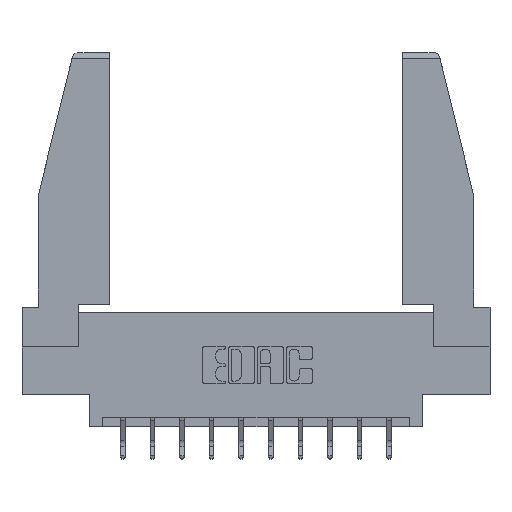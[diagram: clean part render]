
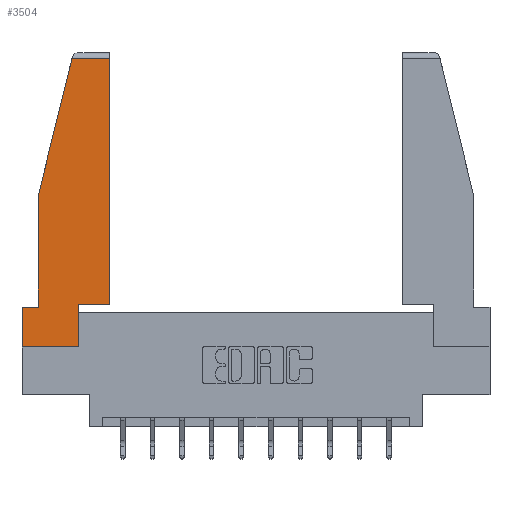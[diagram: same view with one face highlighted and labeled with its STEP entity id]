
A CAD part, top view. The second image highlights one B-rep face of the part: STEP entity #3504.
In plain terms, the highlighted planar face has unit normal (0, 0, 1).
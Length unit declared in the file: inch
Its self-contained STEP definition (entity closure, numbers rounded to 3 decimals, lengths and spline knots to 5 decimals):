
#660 = CARTESIAN_POINT ( 'NONE',  ( 0., 1.52, 0. ) ) ;
#703 = EDGE_CURVE ( 'NONE', #13000, #8001, #8081, .T. ) ;
#913 = CARTESIAN_POINT ( 'NONE',  ( 0.086, 0.21, 0. ) ) ;
#945 = AXIS2_PLACEMENT_3D ( 'NONE', #13486, #1005, #4476 ) ;
#990 = VERTEX_POINT ( 'NONE', #6314 ) ;
#1005 = DIRECTION ( 'NONE',  ( 0., 0., 1. ) ) ;
#1070 = CARTESIAN_POINT ( 'NONE',  ( 0.461, 0.223, 0. ) ) ;
#1220 = DIRECTION ( 'NONE',  ( 1., 0., 0. ) ) ;
#1303 = VECTOR ( 'NONE', #13057, 39.37008 ) ;
#1536 = CARTESIAN_POINT ( 'NONE',  ( 0., 0., 0. ) ) ;
#1809 = LINE ( 'NONE', #13402, #13564 ) ;
#2137 = ORIENTED_EDGE ( 'NONE', *, *, #10737, .T. ) ;
#2247 = ORIENTED_EDGE ( 'NONE', *, *, #11042, .T. ) ;
#2599 = EDGE_CURVE ( 'NONE', #6331, #10988, #8358, .T. ) ;
#3091 = CARTESIAN_POINT ( 'NONE',  ( 0.2636, 1.52, 0. ) ) ;
#3504 = ADVANCED_FACE ( 'NONE', ( #8229 ), #9974, .T. ) ;
#3506 = VERTEX_POINT ( 'NONE', #3091 ) ;
#3553 = DIRECTION ( 'NONE',  ( 0., -1., 0. ) ) ;
#4240 = DIRECTION ( 'NONE',  ( 0., 1., 0. ) ) ;
#4410 = LINE ( 'NONE', #660, #14593 ) ;
#4476 = DIRECTION ( 'NONE',  ( 1., 0., 0. ) ) ;
#4838 = LINE ( 'NONE', #5781, #12177 ) ;
#4849 = LINE ( 'NONE', #7688, #7523 ) ;
#4911 = CARTESIAN_POINT ( 'NONE',  ( 0.297, 0.223, 0. ) ) ;
#5062 = CARTESIAN_POINT ( 'NONE',  ( 0., 0.21, 0. ) ) ;
#5079 = CARTESIAN_POINT ( 'NONE',  ( 0.297, 0., 0. ) ) ;
#5183 = LINE ( 'NONE', #5062, #8581 ) ;
#5534 = VECTOR ( 'NONE', #4240, 39.37008 ) ;
#5781 = CARTESIAN_POINT ( 'NONE',  ( 0.086, 0.8, 0. ) ) ;
#5791 = CARTESIAN_POINT ( 'NONE',  ( 0., 0.21, 0. ) ) ;
#6314 = CARTESIAN_POINT ( 'NONE',  ( 0.461, 1.52, 0. ) ) ;
#6331 = VERTEX_POINT ( 'NONE', #913 ) ;
#6645 = EDGE_CURVE ( 'NONE', #990, #3506, #4410, .T. ) ;
#6963 = DIRECTION ( 'NONE',  ( -1., 0., 0. ) ) ;
#7411 = ORIENTED_EDGE ( 'NONE', *, *, #10278, .T. ) ;
#7464 = VECTOR ( 'NONE', #6963, 39.37008 ) ;
#7523 = VECTOR ( 'NONE', #14342, 39.37008 ) ;
#7688 = CARTESIAN_POINT ( 'NONE',  ( 0.297, 0., 0. ) ) ;
#7828 = ORIENTED_EDGE ( 'NONE', *, *, #703, .T. ) ;
#8001 = VERTEX_POINT ( 'NONE', #1070 ) ;
#8043 = CARTESIAN_POINT ( 'NONE',  ( 0.297, 0.223, 0. ) ) ;
#8050 = LINE ( 'NONE', #11100, #5534 ) ;
#8081 = LINE ( 'NONE', #8043, #9873 ) ;
#8229 = FACE_OUTER_BOUND ( 'NONE', #10277, .T. ) ;
#8358 = LINE ( 'NONE', #5791, #7464 ) ;
#8581 = VECTOR ( 'NONE', #13192, 39.37008 ) ;
#8612 = DIRECTION ( 'NONE',  ( -1., 0., 0. ) ) ;
#8626 = CARTESIAN_POINT ( 'NONE',  ( 0., 0., 0. ) ) ;
#9126 = LINE ( 'NONE', #8626, #1303 ) ;
#9383 = CARTESIAN_POINT ( 'NONE',  ( 0., 0.21, 0. ) ) ;
#9873 = VECTOR ( 'NONE', #1220, 39.37008 ) ;
#9974 = PLANE ( 'NONE',  #945 ) ;
#10083 = VERTEX_POINT ( 'NONE', #11095 ) ;
#10277 = EDGE_LOOP ( 'NONE', ( #2247, #14569, #14651, #2137, #14361, #12227, #13773, #7411, #7828 ) ) ;
#10278 = EDGE_CURVE ( 'NONE', #10771, #13000, #4849, .T. ) ;
#10737 = EDGE_CURVE ( 'NONE', #10083, #6331, #4838, .T. ) ;
#10755 = EDGE_CURVE ( 'NONE', #13445, #10771, #9126, .T. ) ;
#10771 = VERTEX_POINT ( 'NONE', #5079 ) ;
#10970 = EDGE_CURVE ( 'NONE', #10988, #13445, #5183, .T. ) ;
#10988 = VERTEX_POINT ( 'NONE', #9383 ) ;
#11042 = EDGE_CURVE ( 'NONE', #8001, #990, #8050, .T. ) ;
#11095 = CARTESIAN_POINT ( 'NONE',  ( 0.086, 0.8, 0. ) ) ;
#11098 = EDGE_CURVE ( 'NONE', #3506, #10083, #1809, .T. ) ;
#11100 = CARTESIAN_POINT ( 'NONE',  ( 0.461, 0.223, 0. ) ) ;
#12177 = VECTOR ( 'NONE', #3553, 39.37008 ) ;
#12227 = ORIENTED_EDGE ( 'NONE', *, *, #10970, .T. ) ;
#13000 = VERTEX_POINT ( 'NONE', #4911 ) ;
#13057 = DIRECTION ( 'NONE',  ( 1., 0., 0. ) ) ;
#13192 = DIRECTION ( 'NONE',  ( 0., -1., 0. ) ) ;
#13402 = CARTESIAN_POINT ( 'NONE',  ( 0.271, 1.55, 0. ) ) ;
#13445 = VERTEX_POINT ( 'NONE', #1536 ) ;
#13486 = CARTESIAN_POINT ( 'NONE',  ( 0., 0., 0. ) ) ;
#13564 = VECTOR ( 'NONE', #14589, 39.37008 ) ;
#13773 = ORIENTED_EDGE ( 'NONE', *, *, #10755, .T. ) ;
#14342 = DIRECTION ( 'NONE',  ( 0., 1., 0. ) ) ;
#14361 = ORIENTED_EDGE ( 'NONE', *, *, #2599, .T. ) ;
#14569 = ORIENTED_EDGE ( 'NONE', *, *, #6645, .T. ) ;
#14589 = DIRECTION ( 'NONE',  ( -0.239, -0.971, 0. ) ) ;
#14593 = VECTOR ( 'NONE', #8612, 39.37008 ) ;
#14651 = ORIENTED_EDGE ( 'NONE', *, *, #11098, .T. ) ;
